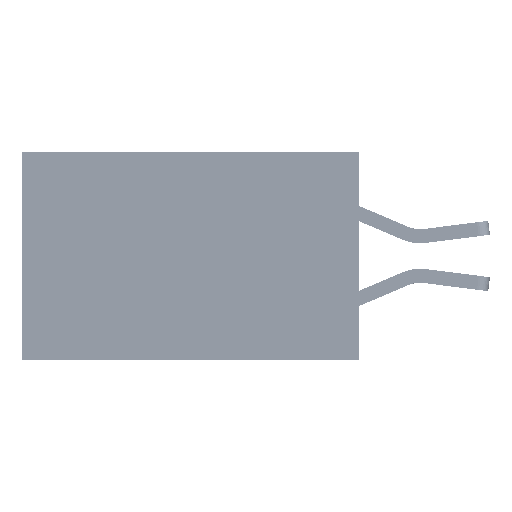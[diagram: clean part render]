
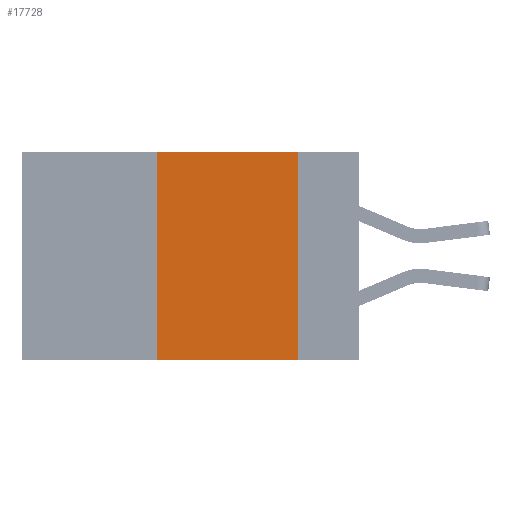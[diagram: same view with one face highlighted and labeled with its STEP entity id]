
A CAD part, left-side view. The second image highlights one B-rep face of the part: STEP entity #17728.
In plain terms, the highlighted planar face has unit normal (-1, 0, 0).
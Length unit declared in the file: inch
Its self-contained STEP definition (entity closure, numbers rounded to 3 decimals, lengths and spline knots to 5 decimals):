
#1176 = AXIS2_PLACEMENT_3D ( 'NONE', #30910, #21373, #24112 ) ;
#1442 = DIRECTION ( 'NONE',  ( 0., 0., 1. ) ) ;
#3452 = DIRECTION ( 'NONE',  ( 0., 0., -1. ) ) ;
#4727 = ORIENTED_EDGE ( 'NONE', *, *, #14500, .F. ) ;
#4733 = CARTESIAN_POINT ( 'NONE',  ( 0., 0.11, 0. ) ) ;
#7531 = VERTEX_POINT ( 'NONE', #4733 ) ;
#7773 = DIRECTION ( 'NONE',  ( 0., -1., 0. ) ) ;
#8424 = VERTEX_POINT ( 'NONE', #34592 ) ;
#8667 = VECTOR ( 'NONE', #7773, 39.37008 ) ;
#9251 = ORIENTED_EDGE ( 'NONE', *, *, #32958, .F. ) ;
#9479 = DIRECTION ( 'NONE',  ( 0., -1., 0. ) ) ;
#11655 = LINE ( 'NONE', #23513, #8667 ) ;
#11833 = CARTESIAN_POINT ( 'NONE',  ( 0., 0.6, 0. ) ) ;
#13732 = ORIENTED_EDGE ( 'NONE', *, *, #29261, .T. ) ;
#14500 = EDGE_CURVE ( 'NONE', #24718, #7531, #15515, .T. ) ;
#15515 = LINE ( 'NONE', #11833, #25953 ) ;
#17728 = ADVANCED_FACE ( 'NONE', ( #21569 ), #30133, .F. ) ;
#18681 = EDGE_LOOP ( 'NONE', ( #9251, #4727, #34562, #13732 ) ) ;
#20782 = CARTESIAN_POINT ( 'NONE',  ( 0., 0.11, -0.37 ) ) ;
#21052 = VERTEX_POINT ( 'NONE', #20782 ) ;
#21373 = DIRECTION ( 'NONE',  ( 1., 0., 0. ) ) ;
#21569 = FACE_OUTER_BOUND ( 'NONE', #18681, .T. ) ;
#21938 = CARTESIAN_POINT ( 'NONE',  ( 0., 0.11, 0. ) ) ;
#23513 = CARTESIAN_POINT ( 'NONE',  ( 0., 0.6, -0.37 ) ) ;
#24112 = DIRECTION ( 'NONE',  ( 0., 0., -1. ) ) ;
#24718 = VERTEX_POINT ( 'NONE', #29226 ) ;
#25953 = VECTOR ( 'NONE', #9479, 39.37008 ) ;
#28755 = VECTOR ( 'NONE', #3452, 39.37008 ) ;
#28855 = EDGE_CURVE ( 'NONE', #8424, #24718, #31988, .T. ) ;
#29226 = CARTESIAN_POINT ( 'NONE',  ( 0., 0.36, 0. ) ) ;
#29261 = EDGE_CURVE ( 'NONE', #8424, #21052, #11655, .T. ) ;
#30108 = LINE ( 'NONE', #21938, #28755 ) ;
#30133 = PLANE ( 'NONE',  #1176 ) ;
#30471 = VECTOR ( 'NONE', #1442, 39.37008 ) ;
#30910 = CARTESIAN_POINT ( 'NONE',  ( 0., 0.6, 0. ) ) ;
#31988 = LINE ( 'NONE', #34501, #30471 ) ;
#32958 = EDGE_CURVE ( 'NONE', #7531, #21052, #30108, .T. ) ;
#34501 = CARTESIAN_POINT ( 'NONE',  ( 0., 0.36, 0. ) ) ;
#34562 = ORIENTED_EDGE ( 'NONE', *, *, #28855, .F. ) ;
#34592 = CARTESIAN_POINT ( 'NONE',  ( 0., 0.36, -0.37 ) ) ;
